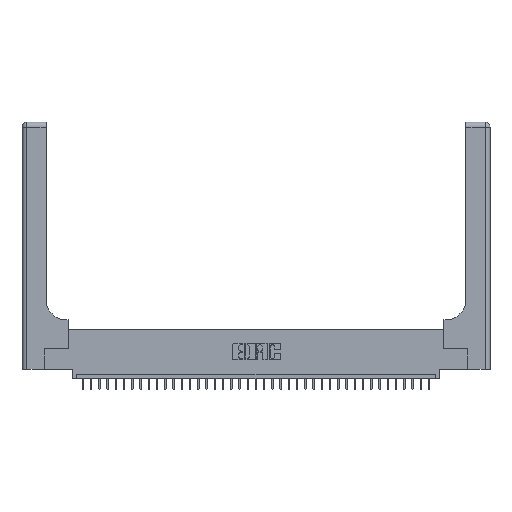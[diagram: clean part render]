
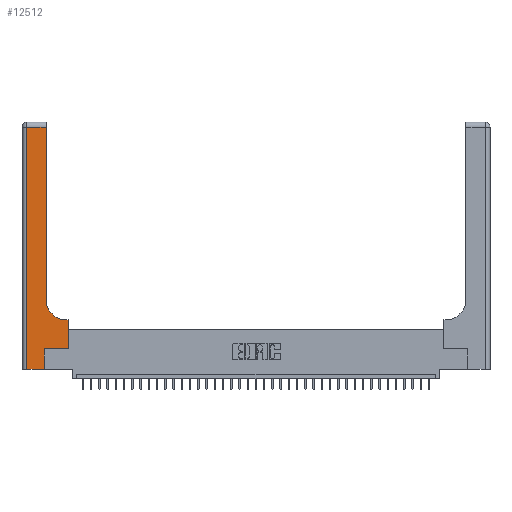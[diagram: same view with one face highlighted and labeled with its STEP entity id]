
A CAD part, top view. The second image highlights one B-rep face of the part: STEP entity #12512.
In plain terms, the highlighted planar face has unit normal (0, 0, 1).
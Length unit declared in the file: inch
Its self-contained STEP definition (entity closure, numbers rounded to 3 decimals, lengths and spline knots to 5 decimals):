
#108 = CARTESIAN_POINT ( 'NONE',  ( 0.06, 0., 0.37 ) ) ;
#401 = CARTESIAN_POINT ( 'NONE',  ( 0.269, 0., 0.37 ) ) ;
#620 = EDGE_CURVE ( 'NONE', #25559, #4371, #24318, .T. ) ;
#1622 = VECTOR ( 'NONE', #23070, 39.37008 ) ;
#1654 = VERTEX_POINT ( 'NONE', #20036 ) ;
#2081 = EDGE_CURVE ( 'NONE', #27991, #2899, #3313, .T. ) ;
#2433 = CARTESIAN_POINT ( 'NONE',  ( 0.2915, 0.6, 0.37 ) ) ;
#2676 = CARTESIAN_POINT ( 'NONE',  ( 0.5415, 0.6, 0.37 ) ) ;
#2899 = VERTEX_POINT ( 'NONE', #2676 ) ;
#3202 = ORIENTED_EDGE ( 'NONE', *, *, #3213, .T. ) ;
#3213 = EDGE_CURVE ( 'NONE', #19520, #12939, #4728, .T. ) ;
#3313 = LINE ( 'NONE', #2433, #18258 ) ;
#3679 = VECTOR ( 'NONE', #25129, 39.37008 ) ;
#4371 = VERTEX_POINT ( 'NONE', #6196 ) ;
#4382 = VERTEX_POINT ( 'NONE', #108 ) ;
#4728 = LINE ( 'NONE', #27966, #3679 ) ;
#4827 = DIRECTION ( 'NONE',  ( 1., 0., 0. ) ) ;
#6108 = DIRECTION ( 'NONE',  ( 0., 1., 0. ) ) ;
#6177 = LINE ( 'NONE', #11526, #20306 ) ;
#6196 = CARTESIAN_POINT ( 'NONE',  ( 0.269, 0.25, 0.37 ) ) ;
#6424 = EDGE_CURVE ( 'NONE', #12939, #4382, #8731, .T. ) ;
#6487 = EDGE_LOOP ( 'NONE', ( #34611, #3202, #15440, #8637, #15202, #14223, #32820, #8680, #7785 ) ) ;
#6965 = AXIS2_PLACEMENT_3D ( 'NONE', #7285, #27686, #30554 ) ;
#7285 = CARTESIAN_POINT ( 'NONE',  ( 0., 3., 0.37 ) ) ;
#7785 = ORIENTED_EDGE ( 'NONE', *, *, #12618, .T. ) ;
#8022 = CARTESIAN_POINT ( 'NONE',  ( 0.269, 0.25, 0.37 ) ) ;
#8123 = VECTOR ( 'NONE', #6108, 39.37008 ) ;
#8373 = CARTESIAN_POINT ( 'NONE',  ( 0., 0., 0.37 ) ) ;
#8637 = ORIENTED_EDGE ( 'NONE', *, *, #20530, .T. ) ;
#8680 = ORIENTED_EDGE ( 'NONE', *, *, #2081, .T. ) ;
#8731 = LINE ( 'NONE', #16075, #14721 ) ;
#10012 = CIRCLE ( 'NONE', #37375, 0.25 ) ;
#10336 = DIRECTION ( 'NONE',  ( 0., -1., 0. ) ) ;
#11056 = LINE ( 'NONE', #8373, #1622 ) ;
#11526 = CARTESIAN_POINT ( 'NONE',  ( 0.5585, 0.25, 0.37 ) ) ;
#11845 = CARTESIAN_POINT ( 'NONE',  ( 0.5585, 0.25, 0.37 ) ) ;
#12068 = DIRECTION ( 'NONE',  ( -1., 0., 0. ) ) ;
#12512 = ADVANCED_FACE ( 'NONE', ( #24478 ), #30733, .F. ) ;
#12618 = EDGE_CURVE ( 'NONE', #2899, #1654, #10012, .T. ) ;
#12856 = CARTESIAN_POINT ( 'NONE',  ( 0.269, 0., 0.37 ) ) ;
#12939 = VERTEX_POINT ( 'NONE', #33172 ) ;
#14223 = ORIENTED_EDGE ( 'NONE', *, *, #19726, .T. ) ;
#14721 = VECTOR ( 'NONE', #10336, 39.37008 ) ;
#14959 = DIRECTION ( 'NONE',  ( 0., 1., 0. ) ) ;
#15202 = ORIENTED_EDGE ( 'NONE', *, *, #620, .T. ) ;
#15440 = ORIENTED_EDGE ( 'NONE', *, *, #6424, .T. ) ;
#15728 = VECTOR ( 'NONE', #24505, 39.37008 ) ;
#16075 = CARTESIAN_POINT ( 'NONE',  ( 0.06, 3., 0.37 ) ) ;
#18258 = VECTOR ( 'NONE', #12068, 39.37008 ) ;
#19520 = VERTEX_POINT ( 'NONE', #29588 ) ;
#19687 = DIRECTION ( 'NONE',  ( 1., 0., 0. ) ) ;
#19726 = EDGE_CURVE ( 'NONE', #4371, #26742, #36582, .T. ) ;
#20036 = CARTESIAN_POINT ( 'NONE',  ( 0.2915, 0.85, 0.37 ) ) ;
#20306 = VECTOR ( 'NONE', #14959, 39.37008 ) ;
#20530 = EDGE_CURVE ( 'NONE', #4382, #25559, #11056, .T. ) ;
#20633 = CARTESIAN_POINT ( 'NONE',  ( 0.2915, 3., 0.37 ) ) ;
#21442 = CARTESIAN_POINT ( 'NONE',  ( 0.5415, 0.85, 0.37 ) ) ;
#23070 = DIRECTION ( 'NONE',  ( 1., 0., 0. ) ) ;
#24318 = LINE ( 'NONE', #12856, #15728 ) ;
#24478 = FACE_OUTER_BOUND ( 'NONE', #6487, .T. ) ;
#24505 = DIRECTION ( 'NONE',  ( 0., 1., 0. ) ) ;
#25129 = DIRECTION ( 'NONE',  ( -1., 0., 0. ) ) ;
#25559 = VERTEX_POINT ( 'NONE', #401 ) ;
#26742 = VERTEX_POINT ( 'NONE', #11845 ) ;
#27686 = DIRECTION ( 'NONE',  ( 0., 0., -1. ) ) ;
#27966 = CARTESIAN_POINT ( 'NONE',  ( 0., 2.94, 0.37 ) ) ;
#27991 = VERTEX_POINT ( 'NONE', #33839 ) ;
#29588 = CARTESIAN_POINT ( 'NONE',  ( 0.2915, 2.94, 0.37 ) ) ;
#29750 = LINE ( 'NONE', #20633, #8123 ) ;
#30554 = DIRECTION ( 'NONE',  ( -1., 0., 0. ) ) ;
#30733 = PLANE ( 'NONE',  #6965 ) ;
#30919 = DIRECTION ( 'NONE',  ( 0., 0., -1. ) ) ;
#31621 = VECTOR ( 'NONE', #19687, 39.37008 ) ;
#31975 = EDGE_CURVE ( 'NONE', #26742, #27991, #6177, .T. ) ;
#32732 = EDGE_CURVE ( 'NONE', #1654, #19520, #29750, .T. ) ;
#32820 = ORIENTED_EDGE ( 'NONE', *, *, #31975, .T. ) ;
#33172 = CARTESIAN_POINT ( 'NONE',  ( 0.06, 2.94, 0.37 ) ) ;
#33839 = CARTESIAN_POINT ( 'NONE',  ( 0.5585, 0.6, 0.37 ) ) ;
#34611 = ORIENTED_EDGE ( 'NONE', *, *, #32732, .T. ) ;
#36582 = LINE ( 'NONE', #8022, #31621 ) ;
#37375 = AXIS2_PLACEMENT_3D ( 'NONE', #21442, #30919, #4827 ) ;
